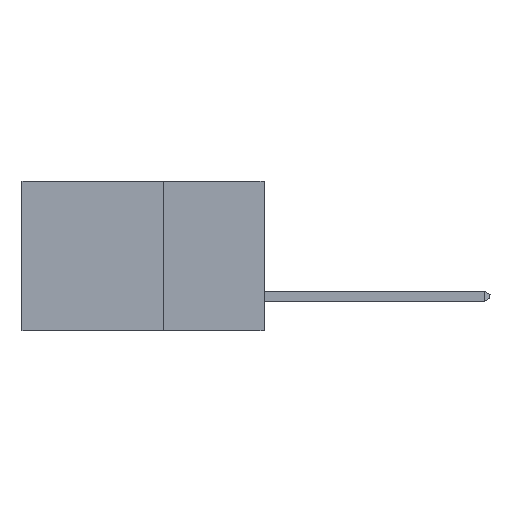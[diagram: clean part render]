
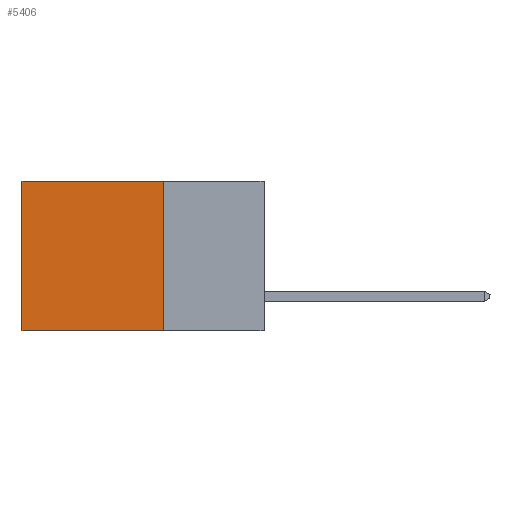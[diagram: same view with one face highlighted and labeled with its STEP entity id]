
A CAD part, left-side view. The second image highlights one B-rep face of the part: STEP entity #5406.
In plain terms, the highlighted planar face has unit normal (-1, 0, 0).
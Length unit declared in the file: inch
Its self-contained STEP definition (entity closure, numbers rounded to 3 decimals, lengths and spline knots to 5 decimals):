
#677 = ORIENTED_EDGE ( 'NONE', *, *, #4958, .T. ) ;
#788 = CARTESIAN_POINT ( 'NONE',  ( 0.298, 0.25, 0. ) ) ;
#865 = EDGE_LOOP ( 'NONE', ( #677, #6780, #8197, #3536 ) ) ;
#1454 = DIRECTION ( 'NONE',  ( 1., 0., 0. ) ) ;
#1598 = LINE ( 'NONE', #6404, #2756 ) ;
#1797 = CARTESIAN_POINT ( 'NONE',  ( 0.298, 0.6, -0.37 ) ) ;
#2598 = DIRECTION ( 'NONE',  ( 0., 1., 0. ) ) ;
#2699 = VERTEX_POINT ( 'NONE', #1797 ) ;
#2756 = VECTOR ( 'NONE', #2598, 39.37008 ) ;
#3536 = ORIENTED_EDGE ( 'NONE', *, *, #5586, .T. ) ;
#4273 = VECTOR ( 'NONE', #6059, 39.37008 ) ;
#4958 = EDGE_CURVE ( 'NONE', #10401, #2699, #6195, .T. ) ;
#5406 = ADVANCED_FACE ( 'NONE', ( #8314 ), #8585, .F. ) ;
#5586 = EDGE_CURVE ( 'NONE', #9126, #10401, #1598, .T. ) ;
#5630 = CARTESIAN_POINT ( 'NONE',  ( 0.298, 0.25, 0. ) ) ;
#6059 = DIRECTION ( 'NONE',  ( 0., 0., -1. ) ) ;
#6195 = LINE ( 'NONE', #13362, #8165 ) ;
#6404 = CARTESIAN_POINT ( 'NONE',  ( 0.298, 0.25, 0. ) ) ;
#6780 = ORIENTED_EDGE ( 'NONE', *, *, #8114, .F. ) ;
#8004 = CARTESIAN_POINT ( 'NONE',  ( 0.298, 0.25, 0. ) ) ;
#8044 = CARTESIAN_POINT ( 'NONE',  ( 0.298, 0.25, -0.37 ) ) ;
#8084 = DIRECTION ( 'NONE',  ( 0., 0., -1. ) ) ;
#8114 = EDGE_CURVE ( 'NONE', #9279, #2699, #11427, .T. ) ;
#8165 = VECTOR ( 'NONE', #8084, 39.37008 ) ;
#8197 = ORIENTED_EDGE ( 'NONE', *, *, #11761, .F. ) ;
#8314 = FACE_OUTER_BOUND ( 'NONE', #865, .T. ) ;
#8585 = PLANE ( 'NONE',  #11141 ) ;
#9126 = VERTEX_POINT ( 'NONE', #8004 ) ;
#9279 = VERTEX_POINT ( 'NONE', #8044 ) ;
#9452 = DIRECTION ( 'NONE',  ( 0., 1., 0. ) ) ;
#9835 = DIRECTION ( 'NONE',  ( 0., 0., -1. ) ) ;
#10401 = VERTEX_POINT ( 'NONE', #11708 ) ;
#11141 = AXIS2_PLACEMENT_3D ( 'NONE', #5630, #1454, #9835 ) ;
#11427 = LINE ( 'NONE', #12513, #12747 ) ;
#11708 = CARTESIAN_POINT ( 'NONE',  ( 0.298, 0.6, 0. ) ) ;
#11761 = EDGE_CURVE ( 'NONE', #9126, #9279, #12232, .T. ) ;
#12232 = LINE ( 'NONE', #788, #4273 ) ;
#12513 = CARTESIAN_POINT ( 'NONE',  ( 0.298, 0.25, -0.37 ) ) ;
#12747 = VECTOR ( 'NONE', #9452, 39.37008 ) ;
#13362 = CARTESIAN_POINT ( 'NONE',  ( 0.298, 0.6, 0. ) ) ;
